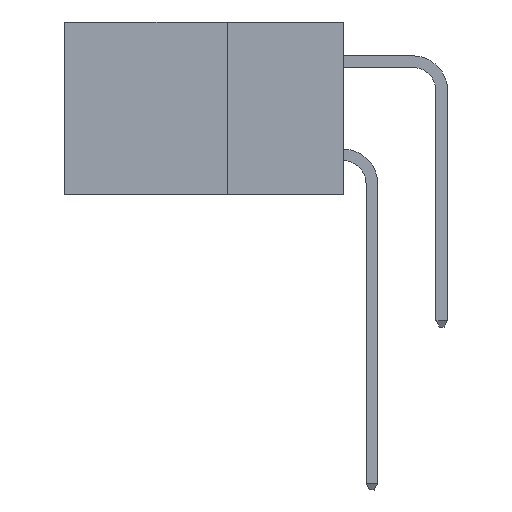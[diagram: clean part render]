
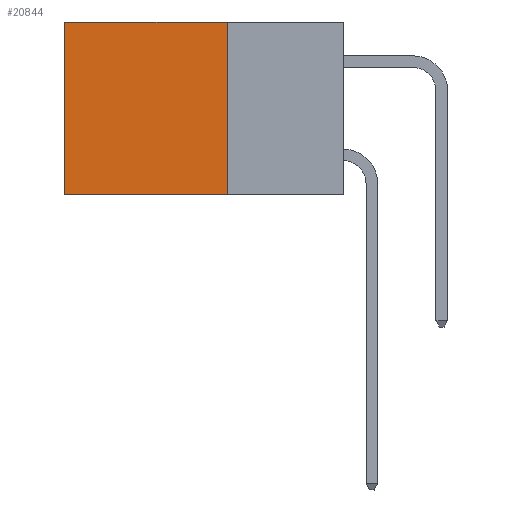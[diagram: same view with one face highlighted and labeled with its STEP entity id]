
A CAD part, left-side view. The second image highlights one B-rep face of the part: STEP entity #20844.
In plain terms, the highlighted planar face has unit normal (-1, 0, 0).
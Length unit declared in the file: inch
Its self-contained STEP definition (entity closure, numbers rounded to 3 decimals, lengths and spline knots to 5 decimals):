
#47 = CARTESIAN_POINT ( 'NONE',  ( 0.298, 0.25, 0. ) ) ;
#427 = ORIENTED_EDGE ( 'NONE', *, *, #6570, .F. ) ;
#1392 = VERTEX_POINT ( 'NONE', #8181 ) ;
#1410 = LINE ( 'NONE', #18661, #6003 ) ;
#1935 = FACE_OUTER_BOUND ( 'NONE', #20933, .T. ) ;
#2056 = CARTESIAN_POINT ( 'NONE',  ( 0.298, 0.25, 0. ) ) ;
#2893 = CARTESIAN_POINT ( 'NONE',  ( 0.298, 0.25, -0.37 ) ) ;
#3214 = EDGE_CURVE ( 'NONE', #13959, #22110, #24609, .T. ) ;
#3784 = LINE ( 'NONE', #2893, #27054 ) ;
#5170 = DIRECTION ( 'NONE',  ( 0., 1., 0. ) ) ;
#6003 = VECTOR ( 'NONE', #11560, 39.37008 ) ;
#6570 = EDGE_CURVE ( 'NONE', #22110, #23630, #3784, .T. ) ;
#6959 = ORIENTED_EDGE ( 'NONE', *, *, #23227, .T. ) ;
#8181 = CARTESIAN_POINT ( 'NONE',  ( 0.298, 0.6, 0. ) ) ;
#9392 = CARTESIAN_POINT ( 'NONE',  ( 0.298, 0.6, -0.37 ) ) ;
#10536 = VECTOR ( 'NONE', #12721, 39.37008 ) ;
#10570 = EDGE_CURVE ( 'NONE', #1392, #23630, #1410, .T. ) ;
#11560 = DIRECTION ( 'NONE',  ( 0., 0., -1. ) ) ;
#11730 = ORIENTED_EDGE ( 'NONE', *, *, #3214, .F. ) ;
#12721 = DIRECTION ( 'NONE',  ( 0., 0., -1. ) ) ;
#13477 = DIRECTION ( 'NONE',  ( 1., 0., 0. ) ) ;
#13569 = DIRECTION ( 'NONE',  ( 0., 1., 0. ) ) ;
#13959 = VERTEX_POINT ( 'NONE', #24039 ) ;
#15827 = DIRECTION ( 'NONE',  ( 0., 0., -1. ) ) ;
#15999 = LINE ( 'NONE', #2056, #25434 ) ;
#17057 = CARTESIAN_POINT ( 'NONE',  ( 0.298, 0.25, 0. ) ) ;
#18661 = CARTESIAN_POINT ( 'NONE',  ( 0.298, 0.6, 0. ) ) ;
#18865 = PLANE ( 'NONE',  #21635 ) ;
#19473 = ORIENTED_EDGE ( 'NONE', *, *, #10570, .T. ) ;
#20844 = ADVANCED_FACE ( 'NONE', ( #1935 ), #18865, .F. ) ;
#20933 = EDGE_LOOP ( 'NONE', ( #19473, #427, #11730, #6959 ) ) ;
#21635 = AXIS2_PLACEMENT_3D ( 'NONE', #47, #13477, #15827 ) ;
#22110 = VERTEX_POINT ( 'NONE', #25299 ) ;
#23227 = EDGE_CURVE ( 'NONE', #13959, #1392, #15999, .T. ) ;
#23630 = VERTEX_POINT ( 'NONE', #9392 ) ;
#24039 = CARTESIAN_POINT ( 'NONE',  ( 0.298, 0.25, 0. ) ) ;
#24609 = LINE ( 'NONE', #17057, #10536 ) ;
#25299 = CARTESIAN_POINT ( 'NONE',  ( 0.298, 0.25, -0.37 ) ) ;
#25434 = VECTOR ( 'NONE', #13569, 39.37008 ) ;
#27054 = VECTOR ( 'NONE', #5170, 39.37008 ) ;
